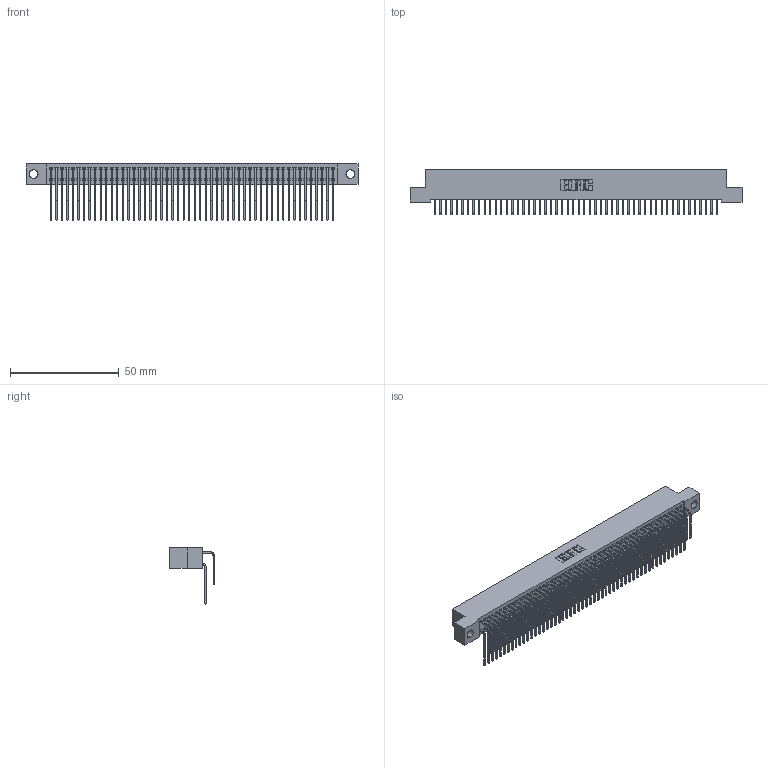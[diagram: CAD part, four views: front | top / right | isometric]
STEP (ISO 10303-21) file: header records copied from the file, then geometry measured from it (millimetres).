
FILE_DESCRIPTION (( 'STEP AP203' ), '1' );
FILE_NAME ('342-104-559-204.STEP', '2019-10-04T18:56:13', ( '' ), ( '' ), 'SwSTEP 2.0', 'SolidWorks 2016', '' );
FILE_SCHEMA (( 'CONFIG_CONTROL_DESIGN' ));
Length unit declared in the file: inch
Products named in the file (4): 345-292-001_559 Tail - 2; 342-104-559-204; 342 Part_.156 TH; 345-292-001_558 559 Tail - 1
Assembly tree (105 placements, depth 2):
  342-104-559-204
    342 Part_.156 TH
    345-292-001_558 559 Tail - 1  x52
    345-292-001_559 Tail - 2  x52
Bounding box: 152.4 x 20.64 x 25.78 mm (x, y, z)
Volume: 14253.4 mm3; surface area: 25985.5 mm2
Topology: 105 solids, 105 shells, 5726 faces, 17043 edges, 11222 vertices
Faces by surface type: plane 4018, cylinder 1708
Entity records: 33815 total; most frequent: CARTESIAN_POINT 5641, ORIENTED_EDGE 5526, DIRECTION 4783, EDGE_CURVE 2763, LINE 2595, VECTOR 2595, VERTEX_POINT 1838, AXIS2_PLACEMENT_3D 1094
